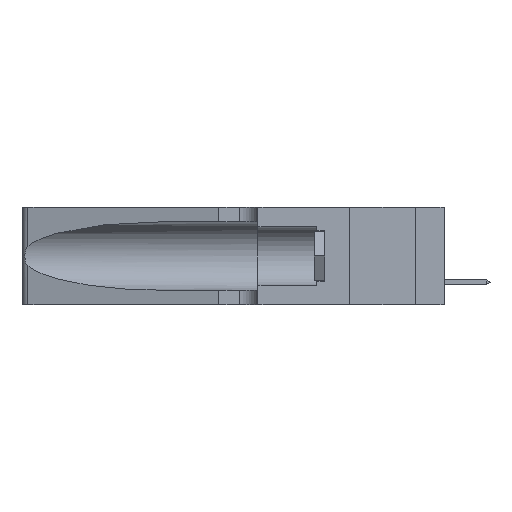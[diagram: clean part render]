
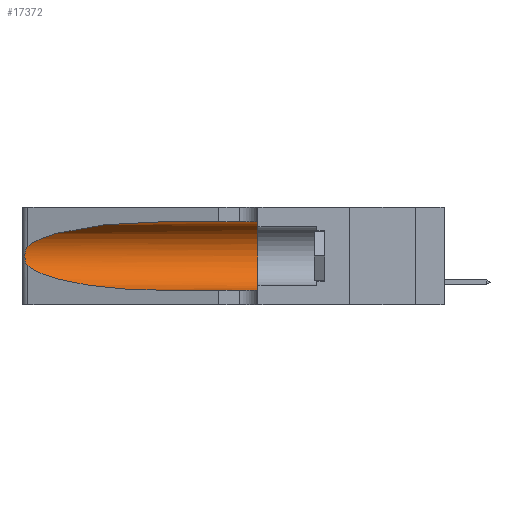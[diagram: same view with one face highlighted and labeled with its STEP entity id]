
A CAD part, left-side view. The second image highlights one B-rep face of the part: STEP entity #17372.
In plain terms, the highlighted cylindrical face has radius 3.308 mm (diameter 6.617 mm), a partial arc.
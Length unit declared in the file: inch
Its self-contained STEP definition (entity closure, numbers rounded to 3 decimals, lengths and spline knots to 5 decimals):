
#758 = CARTESIAN_POINT ( 'NONE',  ( 0.25789, 1.23486, 0.15765 ) ) ;
#955 = CARTESIAN_POINT ( 'NONE',  ( 0.26017, 1.23833, 0.17102 ) ) ;
#1033 = LINE ( 'NONE', #8004, #17216 ) ;
#1155 = CYLINDRICAL_SURFACE ( 'NONE', #14486, 0.13025 ) ;
#1309 = ORIENTED_EDGE ( 'NONE', *, *, #5098, .T. ) ;
#1439 = ORIENTED_EDGE ( 'NONE', *, *, #7761, .T. ) ;
#3253 = VERTEX_POINT ( 'NONE', #9580 ) ;
#3687 = ORIENTED_EDGE ( 'NONE', *, *, #8358, .T. ) ;
#3715 = CARTESIAN_POINT ( 'NONE',  ( 0.25555, 1.22993, 0.14849 ) ) ;
#3791 = VERTEX_POINT ( 'NONE', #8657 ) ;
#3839 = DIRECTION ( 'NONE',  ( 0., -1., 0. ) ) ;
#4708 = LINE ( 'NONE', #9876, #13970 ) ;
#4916 =( BOUNDED_CURVE ( )  B_SPLINE_CURVE ( 3, ( #18354, #12172, #10856, #12422 ),
 .UNSPECIFIED., .F., .T. ) 
 B_SPLINE_CURVE_WITH_KNOTS ( ( 4, 4 ),
 ( 3.44316, 4.71239 ),
 .UNSPECIFIED. ) 
 CURVE ( )  GEOMETRIC_REPRESENTATION_ITEM ( )  RATIONAL_B_SPLINE_CURVE ( ( 1., 0.87, 0.87, 1. ) ) 
 REPRESENTATION_ITEM ( '' )  );
#5098 = EDGE_CURVE ( 'NONE', #3253, #3791, #6363, .T. ) ;
#6140 = AXIS2_PLACEMENT_3D ( 'NONE', #11733, #11795, #8893 ) ;
#6363 =( BOUNDED_CURVE ( )  B_SPLINE_CURVE ( 3, ( #17679, #7593, #13279, #13538 ),
 .UNSPECIFIED., .F., .T. ) 
 B_SPLINE_CURVE_WITH_KNOTS ( ( 4, 4 ),
 ( 1.5708, 2.84003 ),
 .UNSPECIFIED. ) 
 CURVE ( )  GEOMETRIC_REPRESENTATION_ITEM ( )  RATIONAL_B_SPLINE_CURVE ( ( 1., 0.87, 0.87, 1. ) ) 
 REPRESENTATION_ITEM ( '' )  );
#6764 = CARTESIAN_POINT ( 'NONE',  ( 0.25487, 1.22718, 0.14631 ) ) ;
#7562 = DIRECTION ( 'NONE',  ( 0., 0., -1. ) ) ;
#7593 = CARTESIAN_POINT ( 'NONE',  ( 0.18966, 0.96281, 0.31525 ) ) ;
#7761 = EDGE_CURVE ( 'NONE', #3791, #8836, #17511, .T. ) ;
#8004 = CARTESIAN_POINT ( 'NONE',  ( 0.1305, 1.61858, 0.05475 ) ) ;
#8135 = CARTESIAN_POINT ( 'NONE',  ( 0.25639, 1.23184, 0.21858 ) ) ;
#8329 = EDGE_LOOP ( 'NONE', ( #1309, #1439, #17753, #3687, #12024, #18194 ) ) ;
#8358 = EDGE_CURVE ( 'NONE', #14926, #11149, #1033, .T. ) ;
#8657 = CARTESIAN_POINT ( 'NONE',  ( 0.25487, 1.22718, 0.22369 ) ) ;
#8836 = VERTEX_POINT ( 'NONE', #16895 ) ;
#8893 = DIRECTION ( 'NONE',  ( 0., 0., 1. ) ) ;
#9405 = CARTESIAN_POINT ( 'NONE',  ( 0.1305, 0.35, 0.05475 ) ) ;
#9491 = EDGE_CURVE ( 'NONE', #15136, #11149, #12567, .T. ) ;
#9580 = CARTESIAN_POINT ( 'NONE',  ( 0.1305, 0.72297, 0.31525 ) ) ;
#9744 = CARTESIAN_POINT ( 'NONE',  ( 0.25854, 1.2359, 0.20912 ) ) ;
#9806 = CARTESIAN_POINT ( 'NONE',  ( 0.25787, 1.23484, 0.2124 ) ) ;
#9876 = CARTESIAN_POINT ( 'NONE',  ( 0.1305, 1.61858, 0.31525 ) ) ;
#10856 = CARTESIAN_POINT ( 'NONE',  ( 0.18966, 0.96281, 0.05475 ) ) ;
#11116 = CARTESIAN_POINT ( 'NONE',  ( 0.25487, 1.22718, 0.22369 ) ) ;
#11149 = VERTEX_POINT ( 'NONE', #9405 ) ;
#11171 = CARTESIAN_POINT ( 'NONE',  ( 0.26075, 1.23896, 0.19203 ) ) ;
#11236 = CARTESIAN_POINT ( 'NONE',  ( 0.25856, 1.23593, 0.16098 ) ) ;
#11413 = CARTESIAN_POINT ( 'NONE',  ( 0.1305, 0.35, 0.31525 ) ) ;
#11733 = CARTESIAN_POINT ( 'NONE',  ( 0.1305, 0.35, 0.185 ) ) ;
#11795 = DIRECTION ( 'NONE',  ( 0., 1., 0. ) ) ;
#12024 = ORIENTED_EDGE ( 'NONE', *, *, #9491, .F. ) ;
#12172 = CARTESIAN_POINT ( 'NONE',  ( 0.2373, 1.15595, 0.08982 ) ) ;
#12422 = CARTESIAN_POINT ( 'NONE',  ( 0.1305, 0.72297, 0.05475 ) ) ;
#12465 = CARTESIAN_POINT ( 'NONE',  ( 0.1305, 0.72297, 0.05475 ) ) ;
#12567 = CIRCLE ( 'NONE', #6140, 0.13025 ) ;
#12665 = CARTESIAN_POINT ( 'NONE',  ( 0.25639, 1.23186, 0.15144 ) ) ;
#13279 = CARTESIAN_POINT ( 'NONE',  ( 0.2373, 1.15595, 0.28018 ) ) ;
#13538 = CARTESIAN_POINT ( 'NONE',  ( 0.25487, 1.22718, 0.22369 ) ) ;
#13567 = CARTESIAN_POINT ( 'NONE',  ( 0.1305, 1.61858, 0.185 ) ) ;
#13807 = DIRECTION ( 'NONE',  ( 0., -1., 0. ) ) ;
#13970 = VECTOR ( 'NONE', #3839, 39.37008 ) ;
#14486 = AXIS2_PLACEMENT_3D ( 'NONE', #13567, #16247, #7562 ) ;
#14926 = VERTEX_POINT ( 'NONE', #12465 ) ;
#15136 = VERTEX_POINT ( 'NONE', #11413 ) ;
#15905 = EDGE_CURVE ( 'NONE', #3253, #15136, #4708, .T. ) ;
#16247 = DIRECTION ( 'NONE',  ( 0., -1., 0. ) ) ;
#16895 = CARTESIAN_POINT ( 'NONE',  ( 0.25487, 1.22718, 0.14631 ) ) ;
#16965 = CARTESIAN_POINT ( 'NONE',  ( 0.25555, 1.22994, 0.2215 ) ) ;
#17216 = VECTOR ( 'NONE', #13807, 39.37008 ) ;
#17372 = ADVANCED_FACE ( 'NONE', ( #18750 ), #1155, .F. ) ;
#17511 = B_SPLINE_CURVE_WITH_KNOTS ( 'NONE', 3,
 ( #11116, #16965, #8135, #9806, #9744, #18739, #11171, #18598, #955, #11236, #758, #12665, #3715, #6764 ),
 .UNSPECIFIED., .F., .F.,
 ( 4, 2, 2, 2, 2, 2, 4 ),
 ( 0., 0.00027, 0.00053, 0.00107, 0.0016, 0.00187, 0.00214 ),
 .UNSPECIFIED. ) ;
#17525 = EDGE_CURVE ( 'NONE', #8836, #14926, #4916, .T. ) ;
#17679 = CARTESIAN_POINT ( 'NONE',  ( 0.1305, 0.72297, 0.31525 ) ) ;
#17753 = ORIENTED_EDGE ( 'NONE', *, *, #17525, .T. ) ;
#18194 = ORIENTED_EDGE ( 'NONE', *, *, #15905, .F. ) ;
#18354 = CARTESIAN_POINT ( 'NONE',  ( 0.25487, 1.22718, 0.14631 ) ) ;
#18598 = CARTESIAN_POINT ( 'NONE',  ( 0.26075, 1.23896, 0.178 ) ) ;
#18739 = CARTESIAN_POINT ( 'NONE',  ( 0.26018, 1.23835, 0.19895 ) ) ;
#18750 = FACE_OUTER_BOUND ( 'NONE', #8329, .T. ) ;
